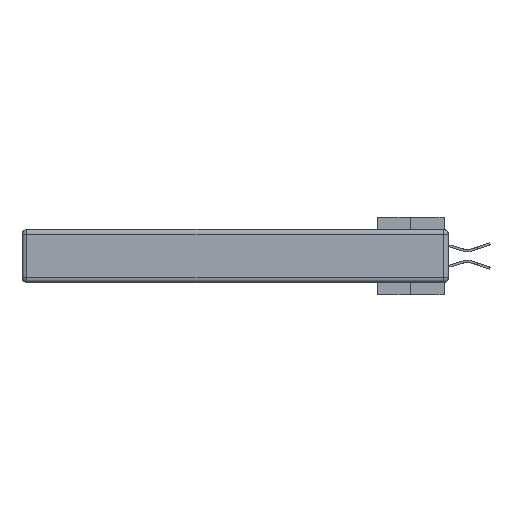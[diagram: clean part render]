
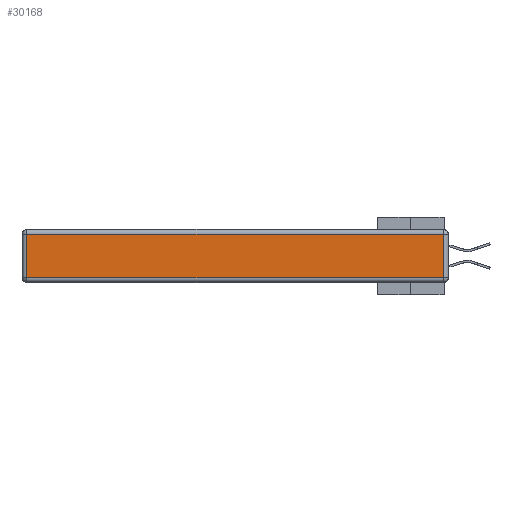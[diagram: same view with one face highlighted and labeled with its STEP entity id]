
A CAD part, left-side view. The second image highlights one B-rep face of the part: STEP entity #30168.
In plain terms, the highlighted planar face has unit normal (-1, 0, 0).
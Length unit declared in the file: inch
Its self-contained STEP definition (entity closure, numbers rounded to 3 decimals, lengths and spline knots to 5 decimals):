
#536 = LINE ( 'NONE', #6721, #8188 ) ;
#1996 = DIRECTION ( 'NONE',  ( 0., 0., 1. ) ) ;
#3026 = CARTESIAN_POINT ( 'NONE',  ( 0., 2.72, -0.03 ) ) ;
#3423 = PLANE ( 'NONE',  #8861 ) ;
#5492 = VERTEX_POINT ( 'NONE', #17413 ) ;
#6721 = CARTESIAN_POINT ( 'NONE',  ( 0., 2.72, -0.343 ) ) ;
#7230 = CARTESIAN_POINT ( 'NONE',  ( 0., 2.75, -0.03 ) ) ;
#8188 = VECTOR ( 'NONE', #29532, 39.37008 ) ;
#8861 = AXIS2_PLACEMENT_3D ( 'NONE', #16228, #29204, #35889 ) ;
#9082 = EDGE_LOOP ( 'NONE', ( #35272, #23377, #33092, #36125 ) ) ;
#9111 = CARTESIAN_POINT ( 'NONE',  ( 0., 0.03, -0.313 ) ) ;
#9542 = VERTEX_POINT ( 'NONE', #3026 ) ;
#13671 = VECTOR ( 'NONE', #16372, 39.37008 ) ;
#14618 = VERTEX_POINT ( 'NONE', #19303 ) ;
#15499 = VERTEX_POINT ( 'NONE', #9111 ) ;
#16228 = CARTESIAN_POINT ( 'NONE',  ( 0., 0., -0.343 ) ) ;
#16372 = DIRECTION ( 'NONE',  ( 0., -1., 0. ) ) ;
#16918 = LINE ( 'NONE', #7230, #22550 ) ;
#17413 = CARTESIAN_POINT ( 'NONE',  ( 0., 0.03, -0.03 ) ) ;
#18968 = LINE ( 'NONE', #41117, #35269 ) ;
#19303 = CARTESIAN_POINT ( 'NONE',  ( 0., 2.72, -0.313 ) ) ;
#22550 = VECTOR ( 'NONE', #26482, 39.37008 ) ;
#23377 = ORIENTED_EDGE ( 'NONE', *, *, #27725, .T. ) ;
#26482 = DIRECTION ( 'NONE',  ( 0., 1., 0. ) ) ;
#27461 = FACE_OUTER_BOUND ( 'NONE', #9082, .T. ) ;
#27725 = EDGE_CURVE ( 'NONE', #15499, #5492, #18968, .T. ) ;
#29044 = EDGE_CURVE ( 'NONE', #9542, #14618, #536, .T. ) ;
#29204 = DIRECTION ( 'NONE',  ( -1., 0., 0. ) ) ;
#29532 = DIRECTION ( 'NONE',  ( 0., 0., -1. ) ) ;
#30168 = ADVANCED_FACE ( 'NONE', ( #27461 ), #3423, .T. ) ;
#30187 = EDGE_CURVE ( 'NONE', #14618, #15499, #37610, .T. ) ;
#32356 = CARTESIAN_POINT ( 'NONE',  ( 0., 0., -0.313 ) ) ;
#33092 = ORIENTED_EDGE ( 'NONE', *, *, #36975, .T. ) ;
#35269 = VECTOR ( 'NONE', #1996, 39.37008 ) ;
#35272 = ORIENTED_EDGE ( 'NONE', *, *, #30187, .T. ) ;
#35889 = DIRECTION ( 'NONE',  ( 0., 0., 1. ) ) ;
#36125 = ORIENTED_EDGE ( 'NONE', *, *, #29044, .T. ) ;
#36975 = EDGE_CURVE ( 'NONE', #5492, #9542, #16918, .T. ) ;
#37610 = LINE ( 'NONE', #32356, #13671 ) ;
#41117 = CARTESIAN_POINT ( 'NONE',  ( 0., 0.03, -0.343 ) ) ;
